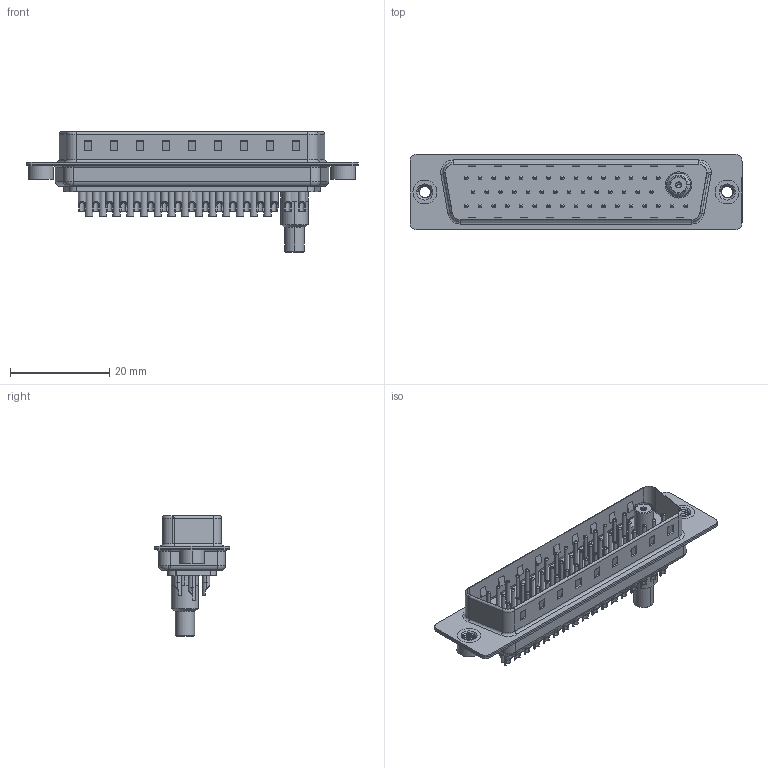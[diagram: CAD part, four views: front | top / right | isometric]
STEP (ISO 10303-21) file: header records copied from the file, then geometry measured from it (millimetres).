
FILE_DESCRIPTION (( 'STEP AP203' ), '1' );
FILE_NAME ('627-47W1622-7NA.STEP', '2019-06-20T16:44:26', ( '' ), ( '' ), 'SwSTEP 2.0', 'SolidWorks 2016', '' );
FILE_SCHEMA (( 'CONFIG_CONTROL_DESIGN' ));
Length unit declared in the file: millimetre
Products named in the file (15): Insulator Socket 2; Locking Collar; 627-47W1622-7NA; Solder Cover; 627Combo Shell Front_50 Contacts; 627Combo Contact Row 1_22; 627Combo Threaded Rivet_A; 627Combo Housing_47W1; 627Combo Contact Row 3_22; Co-Ax Jack Assy_SC; 627Combo Shell Rear_50 Contacts; Insulator Socket; 627Combo Contact Row 2_22L; Co-Ax Jack_Solder Cup Tail; Socket_Solder Cup
Assembly tree (58 placements, depth 3):
  627-47W1622-7NA
    627Combo Housing_47W1
    627Combo Shell Rear_50 Contacts
    627Combo Shell Front_50 Contacts
    627Combo Threaded Rivet_A  x2
    Co-Ax Jack Assy_SC
      Co-Ax Jack_Solder Cup Tail
      Insulator Socket
      Insulator Socket 2
      Locking Collar
      Socket_Solder Cup
      Solder Cover
    627Combo Contact Row 1_22  x15
    627Combo Contact Row 2_22L  x14
    627Combo Contact Row 3_22  x17
Bounding box: 67 x 15.3 x 24.3 mm (x, y, z)
Volume: 4751 mm3; surface area: 12041 mm2
Topology: 57 solids, 57 shells, 2242 faces, 5204 edges, 3184 vertices
Faces by surface type: cylinder 943, plane 657, torus 514, cone 120, bspline 8
Entity records: 33151 total; most frequent: CARTESIAN_POINT 6866, DIRECTION 5324, ORIENTED_EDGE 4552, EDGE_CURVE 2276, AXIS2_PLACEMENT_3D 2119, VERTEX_POINT 1457, EDGE_LOOP 1235, CIRCLE 1099
